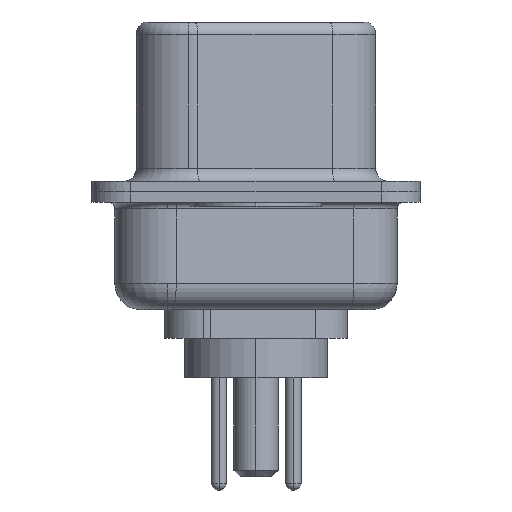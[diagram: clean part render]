
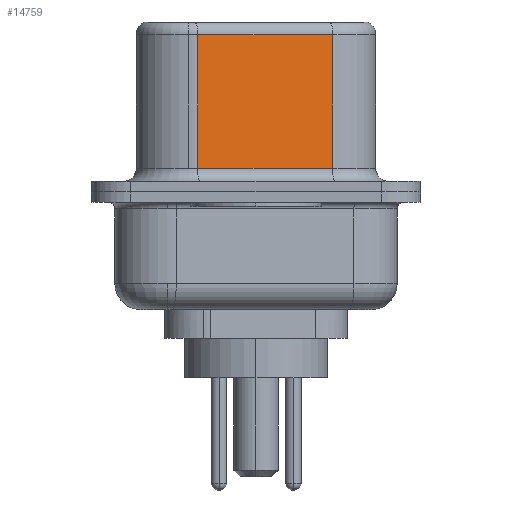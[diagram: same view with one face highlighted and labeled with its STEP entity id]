
A CAD part, left-side view. The second image highlights one B-rep face of the part: STEP entity #14759.
In plain terms, the highlighted planar face has unit normal (-0.985, -0.174, 0).
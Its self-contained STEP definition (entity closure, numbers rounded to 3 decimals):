
#590 = EDGE_CURVE ( 'NONE', #769, #13619, #14005, .T. ) ;
#769 = VERTEX_POINT ( 'NONE', #7202 ) ;
#1015 = CARTESIAN_POINT ( 'NONE',  ( 3.675, 2.233, 0.9 ) ) ;
#2066 = CARTESIAN_POINT ( 'NONE',  ( 4.585, -2.927, 6.52 ) ) ;
#2613 = EDGE_CURVE ( 'NONE', #5565, #10348, #5627, .T. ) ;
#2659 = CARTESIAN_POINT ( 'NONE',  ( 4.585, -2.927, 0.9 ) ) ;
#2718 = LINE ( 'NONE', #8835, #12040 ) ;
#3624 = FACE_OUTER_BOUND ( 'NONE', #5125, .T. ) ;
#3884 = ORIENTED_EDGE ( 'NONE', *, *, #12157, .T. ) ;
#4894 = DIRECTION ( 'NONE',  ( 0., 0., -1. ) ) ;
#4940 = CARTESIAN_POINT ( 'NONE',  ( 4.585, -2.927, 6.52 ) ) ;
#5125 = EDGE_LOOP ( 'NONE', ( #8188, #9497, #13729, #3884 ) ) ;
#5198 = VECTOR ( 'NONE', #9505, 1000. ) ;
#5565 = VERTEX_POINT ( 'NONE', #15537 ) ;
#5594 = LINE ( 'NONE', #5666, #5198 ) ;
#5627 = LINE ( 'NONE', #12963, #12753 ) ;
#5666 = CARTESIAN_POINT ( 'NONE',  ( 4.585, -2.927, 6.02 ) ) ;
#6075 = AXIS2_PLACEMENT_3D ( 'NONE', #4940, #13821, #6247 ) ;
#6247 = DIRECTION ( 'NONE',  ( -0.174, 0.985, 0. ) ) ;
#7202 = CARTESIAN_POINT ( 'NONE',  ( 4.585, -2.927, 6.02 ) ) ;
#8188 = ORIENTED_EDGE ( 'NONE', *, *, #590, .F. ) ;
#8835 = CARTESIAN_POINT ( 'NONE',  ( 4.585, -2.927, 0.9 ) ) ;
#9497 = ORIENTED_EDGE ( 'NONE', *, *, #15118, .T. ) ;
#9505 = DIRECTION ( 'NONE',  ( -0.174, 0.985, 0. ) ) ;
#10348 = VERTEX_POINT ( 'NONE', #1015 ) ;
#10673 = VECTOR ( 'NONE', #4894, 1000. ) ;
#12040 = VECTOR ( 'NONE', #15154, 1000. ) ;
#12157 = EDGE_CURVE ( 'NONE', #10348, #13619, #2718, .T. ) ;
#12753 = VECTOR ( 'NONE', #12908, 1000. ) ;
#12908 = DIRECTION ( 'NONE',  ( 0., 0., -1. ) ) ;
#12963 = CARTESIAN_POINT ( 'NONE',  ( 3.675, 2.233, 6.52 ) ) ;
#13619 = VERTEX_POINT ( 'NONE', #2659 ) ;
#13729 = ORIENTED_EDGE ( 'NONE', *, *, #2613, .T. ) ;
#13821 = DIRECTION ( 'NONE',  ( 0.985, 0.174, 0. ) ) ;
#14005 = LINE ( 'NONE', #2066, #10673 ) ;
#14759 = ADVANCED_FACE ( 'NONE', ( #3624 ), #16338, .F. ) ;
#15118 = EDGE_CURVE ( 'NONE', #769, #5565, #5594, .T. ) ;
#15154 = DIRECTION ( 'NONE',  ( 0.174, -0.985, 0. ) ) ;
#15537 = CARTESIAN_POINT ( 'NONE',  ( 3.675, 2.233, 6.02 ) ) ;
#16338 = PLANE ( 'NONE',  #6075 ) ;
